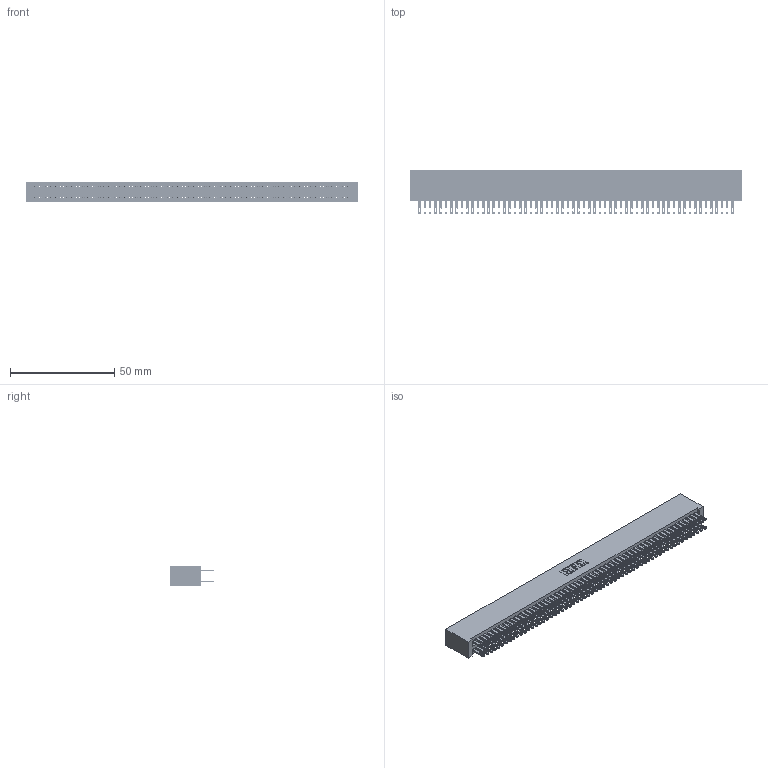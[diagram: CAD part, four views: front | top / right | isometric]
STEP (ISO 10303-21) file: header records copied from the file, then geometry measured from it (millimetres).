
FILE_DESCRIPTION (( 'STEP AP203' ), '1' );
FILE_NAME ('345-120-500-201.STEP', '2019-11-05T23:08:13', ( '' ), ( '' ), 'SwSTEP 2.0', 'SolidWorks 2016', '' );
FILE_SCHEMA (( 'CONFIG_CONTROL_DESIGN' ));
Length unit declared in the file: inch
Products named in the file (3): 345 Part_No Mounting Lugs; 345-120-500-201; 345-292-001_345-293-100
Assembly tree (121 placements, depth 2):
  345-120-500-201
    345 Part_No Mounting Lugs
    345-292-001_345-293-100  x120
Bounding box: 159 x 21.51 x 9.4 mm (x, y, z)
Volume: 16595.5 mm3; surface area: 26406.8 mm2
Topology: 121 solids, 121 shells, 5638 faces, 17237 edges, 11490 vertices
Faces by surface type: plane 3316, cylinder 2322
Entity records: 44307 total; most frequent: CARTESIAN_POINT 7408, ORIENTED_EDGE 7342, DIRECTION 6507, EDGE_CURVE 3671, VECTOR 3303, LINE 3303, VERTEX_POINT 2446, AXIS2_PLACEMENT_3D 1602
